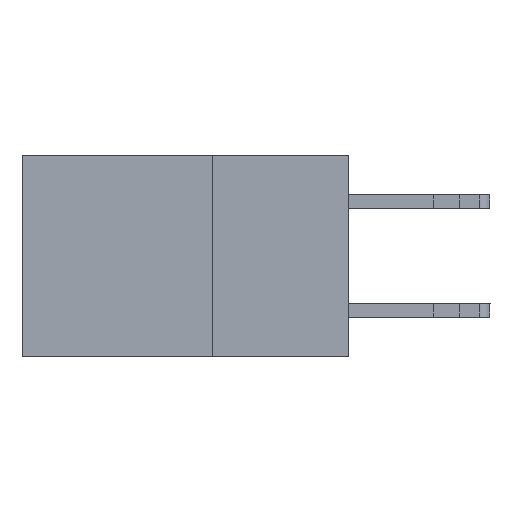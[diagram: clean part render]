
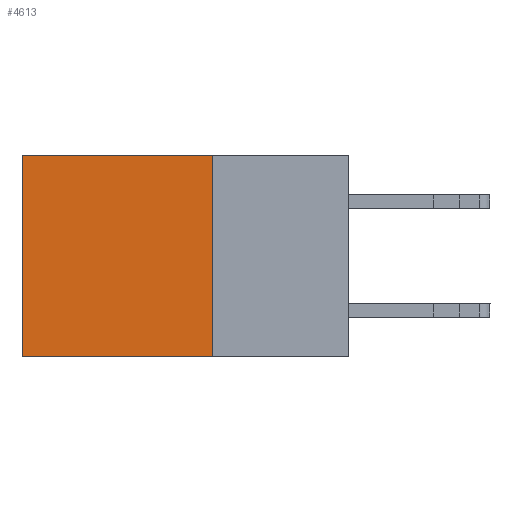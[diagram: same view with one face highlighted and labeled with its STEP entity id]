
A CAD part, left-side view. The second image highlights one B-rep face of the part: STEP entity #4613.
In plain terms, the highlighted planar face has unit normal (-1, 0, 0).
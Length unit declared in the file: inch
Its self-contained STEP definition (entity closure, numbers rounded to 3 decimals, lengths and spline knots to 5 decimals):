
#33 = DIRECTION ( 'NONE',  ( 0., 0., -1. ) ) ;
#122 = EDGE_CURVE ( 'NONE', #9851, #10181, #1534, .T. ) ;
#456 = CARTESIAN_POINT ( 'NONE',  ( 0.2615, 0.25, 0. ) ) ;
#694 = EDGE_CURVE ( 'NONE', #9851, #6111, #13754, .T. ) ;
#1179 = VECTOR ( 'NONE', #8761, 39.37008 ) ;
#1404 = CARTESIAN_POINT ( 'NONE',  ( 0.2615, 0.6, 0. ) ) ;
#1534 = LINE ( 'NONE', #456, #1179 ) ;
#1610 = FACE_OUTER_BOUND ( 'NONE', #3171, .T. ) ;
#3011 = VECTOR ( 'NONE', #9065, 39.37008 ) ;
#3171 = EDGE_LOOP ( 'NONE', ( #5899, #4274, #10596, #3752 ) ) ;
#3218 = CARTESIAN_POINT ( 'NONE',  ( 0.2615, 0.6, -0.37 ) ) ;
#3752 = ORIENTED_EDGE ( 'NONE', *, *, #122, .T. ) ;
#4274 = ORIENTED_EDGE ( 'NONE', *, *, #7039, .F. ) ;
#4613 = ADVANCED_FACE ( 'NONE', ( #1610 ), #6211, .F. ) ;
#5141 = DIRECTION ( 'NONE',  ( 1., 0., 0. ) ) ;
#5283 = VECTOR ( 'NONE', #6207, 39.37008 ) ;
#5899 = ORIENTED_EDGE ( 'NONE', *, *, #8633, .T. ) ;
#6111 = VERTEX_POINT ( 'NONE', #7595 ) ;
#6207 = DIRECTION ( 'NONE',  ( 0., 0., -1. ) ) ;
#6211 = PLANE ( 'NONE',  #9981 ) ;
#6462 = VECTOR ( 'NONE', #33, 39.37008 ) ;
#6857 = CARTESIAN_POINT ( 'NONE',  ( 0.2615, 0.6, -0.37 ) ) ;
#7039 = EDGE_CURVE ( 'NONE', #6111, #11634, #8950, .T. ) ;
#7595 = CARTESIAN_POINT ( 'NONE',  ( 0.2615, 0.25, -0.37 ) ) ;
#7964 = CARTESIAN_POINT ( 'NONE',  ( 0.2615, 0.25, -0.37 ) ) ;
#8440 = CARTESIAN_POINT ( 'NONE',  ( 0.2615, 0.25, -0.37 ) ) ;
#8633 = EDGE_CURVE ( 'NONE', #10181, #11634, #12011, .T. ) ;
#8761 = DIRECTION ( 'NONE',  ( 0., 1., 0. ) ) ;
#8950 = LINE ( 'NONE', #7964, #3011 ) ;
#9065 = DIRECTION ( 'NONE',  ( 0., 1., 0. ) ) ;
#9851 = VERTEX_POINT ( 'NONE', #12976 ) ;
#9981 = AXIS2_PLACEMENT_3D ( 'NONE', #11783, #5141, #12897 ) ;
#10181 = VERTEX_POINT ( 'NONE', #1404 ) ;
#10596 = ORIENTED_EDGE ( 'NONE', *, *, #694, .F. ) ;
#11634 = VERTEX_POINT ( 'NONE', #6857 ) ;
#11783 = CARTESIAN_POINT ( 'NONE',  ( 0.2615, 0.25, -0.37 ) ) ;
#12011 = LINE ( 'NONE', #3218, #6462 ) ;
#12897 = DIRECTION ( 'NONE',  ( 0., 0., -1. ) ) ;
#12976 = CARTESIAN_POINT ( 'NONE',  ( 0.2615, 0.25, 0. ) ) ;
#13754 = LINE ( 'NONE', #8440, #5283 ) ;
